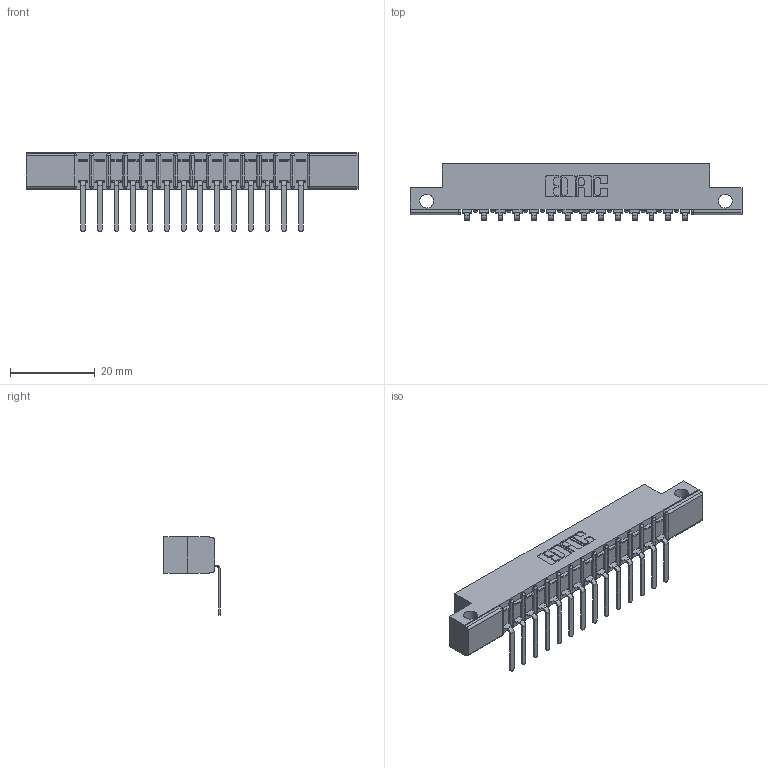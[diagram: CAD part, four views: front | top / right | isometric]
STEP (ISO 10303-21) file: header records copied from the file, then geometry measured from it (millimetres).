
FILE_DESCRIPTION (( 'STEP AP203' ), '1' );
FILE_NAME ('307-014-557-112.STEP', '2018-08-03T01:03:46', ( '' ), ( '' ), 'SwSTEP 2.0', 'SolidWorks 2016', '' );
FILE_SCHEMA (( 'CONFIG_CONTROL_DESIGN' ));
Length unit declared in the file: inch
Products named in the file (3): 307 Part_.128 Dia Side Mounting Holes; 307-290-002_557; 307-014-557-112
Assembly tree (15 placements, depth 2):
  307-014-557-112
    307 Part_.128 Dia Side Mounting Holes
    307-290-002_557  x14
Bounding box: 78.49 x 13.32 x 18.67 mm (x, y, z)
Volume: 5139.2 mm3; surface area: 8995.8 mm2
Topology: 15 solids, 15 shells, 1225 faces, 3739 edges, 2450 vertices
Faces by surface type: plane 728, cylinder 467, sphere 30
Entity records: 16310 total; most frequent: CARTESIAN_POINT 2748, ORIENTED_EDGE 2738, DIRECTION 2683, EDGE_CURVE 1369, LINE 1033, VECTOR 1033, VERTEX_POINT 890, AXIS2_PLACEMENT_3D 825
